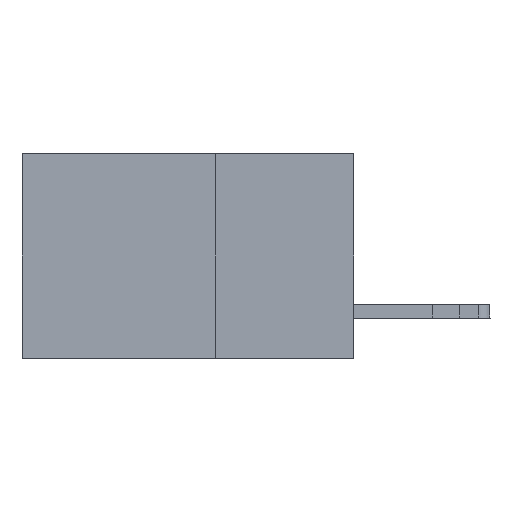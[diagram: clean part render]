
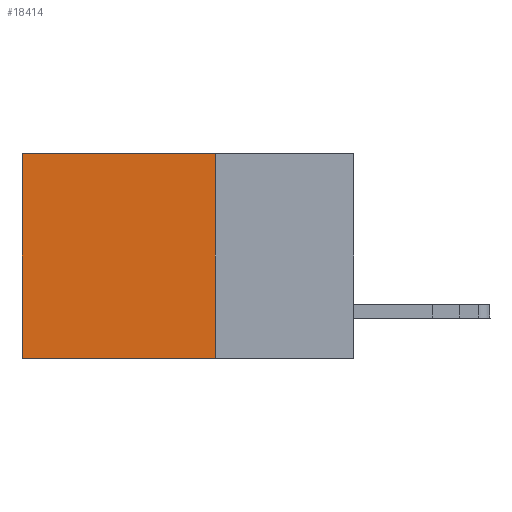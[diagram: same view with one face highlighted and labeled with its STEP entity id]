
A CAD part, left-side view. The second image highlights one B-rep face of the part: STEP entity #18414.
In plain terms, the highlighted planar face has unit normal (-1, 0, 0).
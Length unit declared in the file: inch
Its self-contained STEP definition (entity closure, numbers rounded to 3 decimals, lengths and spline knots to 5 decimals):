
#598 = CARTESIAN_POINT ( 'NONE',  ( 0.2875, 0.25, -0.37 ) ) ;
#1351 = EDGE_LOOP ( 'NONE', ( #14796, #15809, #29419, #16390 ) ) ;
#3410 = VERTEX_POINT ( 'NONE', #12954 ) ;
#4421 = CARTESIAN_POINT ( 'NONE',  ( 0.2875, 0.25, 0. ) ) ;
#4827 = VERTEX_POINT ( 'NONE', #24659 ) ;
#4944 = EDGE_CURVE ( 'NONE', #18184, #3410, #10523, .T. ) ;
#6431 = DIRECTION ( 'NONE',  ( 0., 0., -1. ) ) ;
#6737 = DIRECTION ( 'NONE',  ( 1., 0., 0. ) ) ;
#8237 = DIRECTION ( 'NONE',  ( 0., 1., 0. ) ) ;
#9141 = LINE ( 'NONE', #11723, #28164 ) ;
#9296 = LINE ( 'NONE', #4421, #25606 ) ;
#10363 = CARTESIAN_POINT ( 'NONE',  ( 0.2875, 0.25, -0.37 ) ) ;
#10523 = LINE ( 'NONE', #10363, #20631 ) ;
#11723 = CARTESIAN_POINT ( 'NONE',  ( 0.2875, 0.25, 0. ) ) ;
#12298 = VERTEX_POINT ( 'NONE', #18253 ) ;
#12377 = LINE ( 'NONE', #22291, #21967 ) ;
#12611 = EDGE_CURVE ( 'NONE', #12298, #3410, #12377, .T. ) ;
#12954 = CARTESIAN_POINT ( 'NONE',  ( 0.2875, 0.6, -0.37 ) ) ;
#13541 = DIRECTION ( 'NONE',  ( 0., 0., -1. ) ) ;
#14537 = AXIS2_PLACEMENT_3D ( 'NONE', #28667, #6737, #6431 ) ;
#14796 = ORIENTED_EDGE ( 'NONE', *, *, #12611, .T. ) ;
#15809 = ORIENTED_EDGE ( 'NONE', *, *, #4944, .F. ) ;
#16390 = ORIENTED_EDGE ( 'NONE', *, *, #30593, .T. ) ;
#18184 = VERTEX_POINT ( 'NONE', #598 ) ;
#18253 = CARTESIAN_POINT ( 'NONE',  ( 0.2875, 0.6, 0. ) ) ;
#18414 = ADVANCED_FACE ( 'NONE', ( #26393 ), #28507, .F. ) ;
#20631 = VECTOR ( 'NONE', #8237, 39.37008 ) ;
#21967 = VECTOR ( 'NONE', #25059, 39.37008 ) ;
#22291 = CARTESIAN_POINT ( 'NONE',  ( 0.2875, 0.6, 0. ) ) ;
#22436 = EDGE_CURVE ( 'NONE', #4827, #18184, #9141, .T. ) ;
#24659 = CARTESIAN_POINT ( 'NONE',  ( 0.2875, 0.25, 0. ) ) ;
#25059 = DIRECTION ( 'NONE',  ( 0., 0., -1. ) ) ;
#25606 = VECTOR ( 'NONE', #29264, 39.37008 ) ;
#26393 = FACE_OUTER_BOUND ( 'NONE', #1351, .T. ) ;
#28164 = VECTOR ( 'NONE', #13541, 39.37008 ) ;
#28507 = PLANE ( 'NONE',  #14537 ) ;
#28667 = CARTESIAN_POINT ( 'NONE',  ( 0.2875, 0.25, 0. ) ) ;
#29264 = DIRECTION ( 'NONE',  ( 0., 1., 0. ) ) ;
#29419 = ORIENTED_EDGE ( 'NONE', *, *, #22436, .F. ) ;
#30593 = EDGE_CURVE ( 'NONE', #4827, #12298, #9296, .T. ) ;
